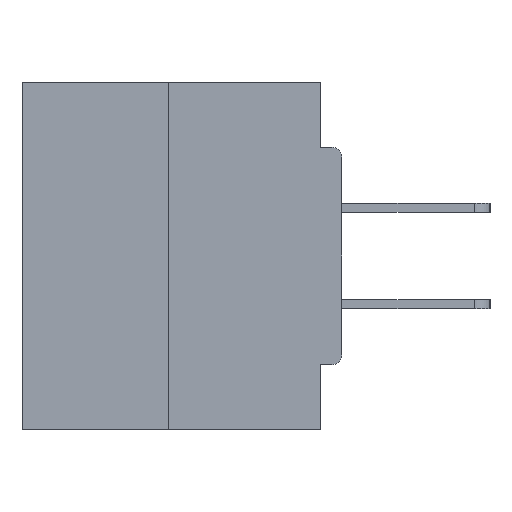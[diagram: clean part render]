
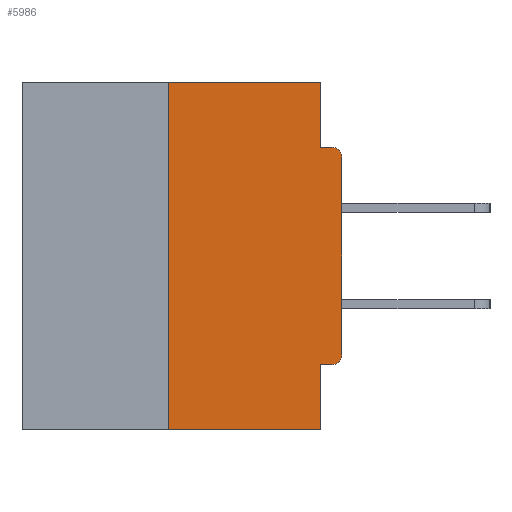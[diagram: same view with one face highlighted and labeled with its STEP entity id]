
A CAD part, left-side view. The second image highlights one B-rep face of the part: STEP entity #5986.
In plain terms, the highlighted planar face has unit normal (-1, 0, 0).
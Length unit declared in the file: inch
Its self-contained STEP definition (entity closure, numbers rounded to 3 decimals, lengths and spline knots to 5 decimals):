
#923 = ORIENTED_EDGE ( 'NONE', *, *, #28653, .F. ) ;
#1034 = DIRECTION ( 'NONE',  ( -1., 0., 0. ) ) ;
#2540 = LINE ( 'NONE', #40417, #5107 ) ;
#3219 = CARTESIAN_POINT ( 'NONE',  ( 0., 0.46, 0. ) ) ;
#3772 = LINE ( 'NONE', #26762, #16626 ) ;
#5107 = VECTOR ( 'NONE', #16731, 39.37008 ) ;
#5203 = EDGE_CURVE ( 'NONE', #33396, #21695, #5512, .T. ) ;
#5381 = CARTESIAN_POINT ( 'NONE',  ( 0., 0., -0.0935 ) ) ;
#5512 = CIRCLE ( 'NONE', #37516, 0.015 ) ;
#5789 = ORIENTED_EDGE ( 'NONE', *, *, #11958, .T. ) ;
#5940 = EDGE_CURVE ( 'NONE', #28389, #12917, #39816, .T. ) ;
#5986 = ADVANCED_FACE ( 'NONE', ( #21412 ), #38922, .F. ) ;
#6117 = ORIENTED_EDGE ( 'NONE', *, *, #12853, .F. ) ;
#6231 = VECTOR ( 'NONE', #16469, 39.37008 ) ;
#6453 = CARTESIAN_POINT ( 'NONE',  ( 0., 0.031, -0.0935 ) ) ;
#8006 = CARTESIAN_POINT ( 'NONE',  ( 0., 0.25, -0.5 ) ) ;
#8173 = VERTEX_POINT ( 'NONE', #36580 ) ;
#8868 = VERTEX_POINT ( 'NONE', #27613 ) ;
#9411 = VECTOR ( 'NONE', #19484, 39.37008 ) ;
#9548 = CARTESIAN_POINT ( 'NONE',  ( 0., 0.031, -0.5 ) ) ;
#9932 = DIRECTION ( 'NONE',  ( 0., 0., -1. ) ) ;
#10046 = VERTEX_POINT ( 'NONE', #36124 ) ;
#10958 = ORIENTED_EDGE ( 'NONE', *, *, #21350, .T. ) ;
#11425 = CARTESIAN_POINT ( 'NONE',  ( 0., 0.031, -0.4065 ) ) ;
#11958 = EDGE_CURVE ( 'NONE', #14246, #8868, #40493, .T. ) ;
#11988 = EDGE_CURVE ( 'NONE', #8868, #33396, #2540, .T. ) ;
#12240 = CARTESIAN_POINT ( 'NONE',  ( 0., 0., -0.1085 ) ) ;
#12604 = LINE ( 'NONE', #5381, #37736 ) ;
#12853 = EDGE_CURVE ( 'NONE', #14246, #28389, #40816, .T. ) ;
#12917 = VERTEX_POINT ( 'NONE', #17404 ) ;
#13515 = LINE ( 'NONE', #25760, #9411 ) ;
#13600 = DIRECTION ( 'NONE',  ( 0., 0., -1. ) ) ;
#14060 = EDGE_LOOP ( 'NONE', ( #923, #36643, #10958, #32821, #6117, #5789, #25578, #40373, #30347, #16329 ) ) ;
#14100 = EDGE_CURVE ( 'NONE', #27922, #10046, #13515, .T. ) ;
#14246 = VERTEX_POINT ( 'NONE', #29902 ) ;
#16176 = DIRECTION ( 'NONE',  ( 0., -1., 0. ) ) ;
#16190 = DIRECTION ( 'NONE',  ( 1., 0., 0. ) ) ;
#16329 = ORIENTED_EDGE ( 'NONE', *, *, #20466, .F. ) ;
#16469 = DIRECTION ( 'NONE',  ( 0., -1., 0. ) ) ;
#16626 = VECTOR ( 'NONE', #13600, 39.37008 ) ;
#16731 = DIRECTION ( 'NONE',  ( 0., 0., 1. ) ) ;
#17404 = CARTESIAN_POINT ( 'NONE',  ( 0., 0.031, -0.5 ) ) ;
#18738 = DIRECTION ( 'NONE',  ( 0., -1., 0. ) ) ;
#19346 = CARTESIAN_POINT ( 'NONE',  ( 0., 0.46, 0. ) ) ;
#19484 = DIRECTION ( 'NONE',  ( 0., 0., 1. ) ) ;
#19592 = CARTESIAN_POINT ( 'NONE',  ( 0., 0.46, -0.5 ) ) ;
#19888 = VECTOR ( 'NONE', #35922, 39.37008 ) ;
#20466 = EDGE_CURVE ( 'NONE', #8173, #33862, #3772, .T. ) ;
#21020 = CARTESIAN_POINT ( 'NONE',  ( 0., 0.015, -0.0935 ) ) ;
#21350 = EDGE_CURVE ( 'NONE', #27922, #12917, #34935, .T. ) ;
#21412 = FACE_OUTER_BOUND ( 'NONE', #14060, .T. ) ;
#21695 = VERTEX_POINT ( 'NONE', #21020 ) ;
#23843 = CARTESIAN_POINT ( 'NONE',  ( 0., 0.015, -0.1085 ) ) ;
#25499 = CARTESIAN_POINT ( 'NONE',  ( 0., 0., -0.4065 ) ) ;
#25578 = ORIENTED_EDGE ( 'NONE', *, *, #11988, .T. ) ;
#25760 = CARTESIAN_POINT ( 'NONE',  ( 0., 0.25, 0. ) ) ;
#26762 = CARTESIAN_POINT ( 'NONE',  ( 0., 0.031, 0. ) ) ;
#26816 = DIRECTION ( 'NONE',  ( 0., 0., -1. ) ) ;
#26899 = DIRECTION ( 'NONE',  ( 0., 0., -1. ) ) ;
#27613 = CARTESIAN_POINT ( 'NONE',  ( 0., 0., -0.3915 ) ) ;
#27922 = VERTEX_POINT ( 'NONE', #8006 ) ;
#28389 = VERTEX_POINT ( 'NONE', #11425 ) ;
#28653 = EDGE_CURVE ( 'NONE', #10046, #8173, #35815, .T. ) ;
#29147 = VECTOR ( 'NONE', #16176, 39.37008 ) ;
#29902 = CARTESIAN_POINT ( 'NONE',  ( 0., 0.015, -0.4065 ) ) ;
#30347 = ORIENTED_EDGE ( 'NONE', *, *, #30454, .F. ) ;
#30454 = EDGE_CURVE ( 'NONE', #33862, #21695, #12604, .T. ) ;
#32200 = DIRECTION ( 'NONE',  ( 0., 1., 0. ) ) ;
#32712 = CARTESIAN_POINT ( 'NONE',  ( 0., 0.015, -0.3915 ) ) ;
#32821 = ORIENTED_EDGE ( 'NONE', *, *, #5940, .F. ) ;
#33396 = VERTEX_POINT ( 'NONE', #12240 ) ;
#33862 = VERTEX_POINT ( 'NONE', #6453 ) ;
#34935 = LINE ( 'NONE', #19592, #6231 ) ;
#35815 = LINE ( 'NONE', #3219, #29147 ) ;
#35922 = DIRECTION ( 'NONE',  ( 0., 0., -1. ) ) ;
#36124 = CARTESIAN_POINT ( 'NONE',  ( 0., 0.25, 0. ) ) ;
#36580 = CARTESIAN_POINT ( 'NONE',  ( 0., 0.031, 0. ) ) ;
#36643 = ORIENTED_EDGE ( 'NONE', *, *, #14100, .F. ) ;
#37516 = AXIS2_PLACEMENT_3D ( 'NONE', #23843, #1034, #26816 ) ;
#37736 = VECTOR ( 'NONE', #18738, 39.37008 ) ;
#38114 = AXIS2_PLACEMENT_3D ( 'NONE', #32712, #39599, #9932 ) ;
#38679 = AXIS2_PLACEMENT_3D ( 'NONE', #19346, #16190, #26899 ) ;
#38922 = PLANE ( 'NONE',  #38679 ) ;
#39599 = DIRECTION ( 'NONE',  ( -1., 0., 0. ) ) ;
#39816 = LINE ( 'NONE', #9548, #19888 ) ;
#40373 = ORIENTED_EDGE ( 'NONE', *, *, #5203, .T. ) ;
#40417 = CARTESIAN_POINT ( 'NONE',  ( 0., 0., 0. ) ) ;
#40493 = CIRCLE ( 'NONE', #38114, 0.015 ) ;
#40816 = LINE ( 'NONE', #25499, #41847 ) ;
#41847 = VECTOR ( 'NONE', #32200, 39.37008 ) ;
